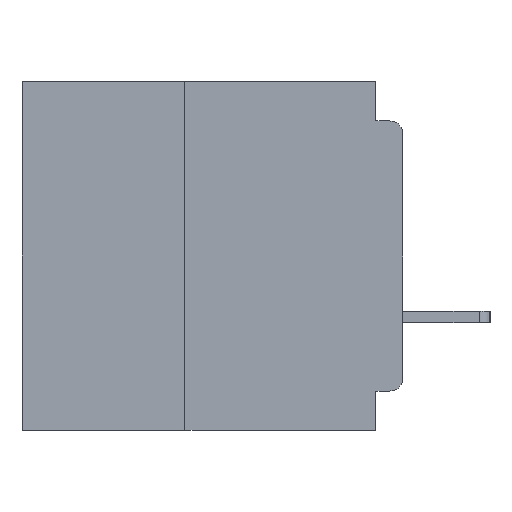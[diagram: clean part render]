
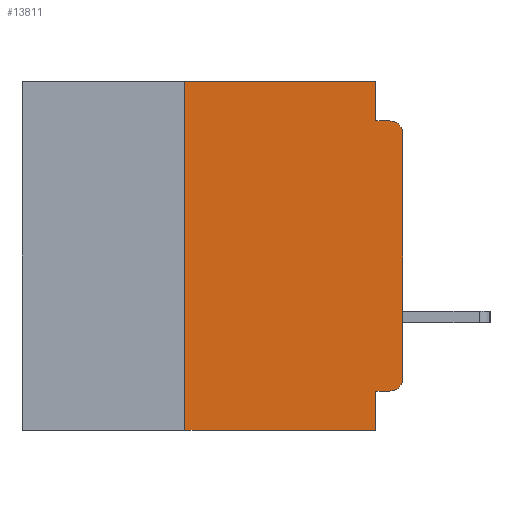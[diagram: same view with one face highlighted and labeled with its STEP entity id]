
A CAD part, left-side view. The second image highlights one B-rep face of the part: STEP entity #13811.
In plain terms, the highlighted planar face has unit normal (-1, 0, 0).
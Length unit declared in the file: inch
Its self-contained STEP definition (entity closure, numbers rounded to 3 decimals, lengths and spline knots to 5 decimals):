
#309 = EDGE_CURVE ( 'NONE', #36454, #38292, #2453, .T. ) ;
#1928 = LINE ( 'NONE', #43107, #9298 ) ;
#2356 = CARTESIAN_POINT ( 'NONE',  ( 0., 0.031, 0. ) ) ;
#2453 = LINE ( 'NONE', #35825, #27884 ) ;
#3500 = DIRECTION ( 'NONE',  ( 0., 0., 1. ) ) ;
#4695 = ORIENTED_EDGE ( 'NONE', *, *, #309, .F. ) ;
#4948 = AXIS2_PLACEMENT_3D ( 'NONE', #11540, #36747, #15153 ) ;
#6119 = AXIS2_PLACEMENT_3D ( 'NONE', #19516, #44719, #23129 ) ;
#6169 = LINE ( 'NONE', #45189, #42315 ) ;
#8141 = CARTESIAN_POINT ( 'NONE',  ( 0., 0.437, -0.4 ) ) ;
#8371 = CARTESIAN_POINT ( 'NONE',  ( 0., 0.031, 0. ) ) ;
#8539 = VECTOR ( 'NONE', #34878, 39.37008 ) ;
#8747 = LINE ( 'NONE', #31282, #17254 ) ;
#9298 = VECTOR ( 'NONE', #3500, 39.37008 ) ;
#9347 = CARTESIAN_POINT ( 'NONE',  ( 0., 0.031, -0.045 ) ) ;
#10352 = LINE ( 'NONE', #8141, #28379 ) ;
#11044 = ORIENTED_EDGE ( 'NONE', *, *, #30380, .T. ) ;
#11198 = EDGE_CURVE ( 'NONE', #35608, #17319, #27740, .T. ) ;
#11540 = CARTESIAN_POINT ( 'NONE',  ( 0., 0.015, -0.06 ) ) ;
#11821 = DIRECTION ( 'NONE',  ( 0., -1., 0. ) ) ;
#12366 = EDGE_LOOP ( 'NONE', ( #11044, #24002, #21811, #13815, #34124, #15558, #24963, #35182, #4695, #12725 ) ) ;
#12725 = ORIENTED_EDGE ( 'NONE', *, *, #41138, .T. ) ;
#13356 = DIRECTION ( 'NONE',  ( 0., -1., 0. ) ) ;
#13811 = ADVANCED_FACE ( 'NONE', ( #39879 ), #14224, .F. ) ;
#13815 = ORIENTED_EDGE ( 'NONE', *, *, #11198, .F. ) ;
#14224 = PLANE ( 'NONE',  #33964 ) ;
#14741 = CIRCLE ( 'NONE', #4948, 0.015 ) ;
#15153 = DIRECTION ( 'NONE',  ( 0., 0., -1. ) ) ;
#15558 = ORIENTED_EDGE ( 'NONE', *, *, #16684, .F. ) ;
#16469 = EDGE_CURVE ( 'NONE', #34442, #16898, #10352, .T. ) ;
#16545 = CIRCLE ( 'NONE', #6119, 0.015 ) ;
#16684 = EDGE_CURVE ( 'NONE', #34442, #17549, #6169, .T. ) ;
#16898 = VERTEX_POINT ( 'NONE', #31930 ) ;
#17254 = VECTOR ( 'NONE', #13356, 39.37008 ) ;
#17319 = VERTEX_POINT ( 'NONE', #9347 ) ;
#17549 = VERTEX_POINT ( 'NONE', #28563 ) ;
#17862 = DIRECTION ( 'NONE',  ( 0., 0., -1. ) ) ;
#18451 = VECTOR ( 'NONE', #18762, 39.37008 ) ;
#18762 = DIRECTION ( 'NONE',  ( 0., 0., -1. ) ) ;
#19140 = VECTOR ( 'NONE', #30762, 39.37008 ) ;
#19516 = CARTESIAN_POINT ( 'NONE',  ( 0., 0.015, -0.34 ) ) ;
#19777 = VERTEX_POINT ( 'NONE', #31505 ) ;
#21811 = ORIENTED_EDGE ( 'NONE', *, *, #30209, .F. ) ;
#22001 = VERTEX_POINT ( 'NONE', #29022 ) ;
#23129 = DIRECTION ( 'NONE',  ( 0., 0., -1. ) ) ;
#24002 = ORIENTED_EDGE ( 'NONE', *, *, #42208, .T. ) ;
#24963 = ORIENTED_EDGE ( 'NONE', *, *, #16469, .T. ) ;
#27740 = LINE ( 'NONE', #2356, #8539 ) ;
#27884 = VECTOR ( 'NONE', #35764, 39.37008 ) ;
#28379 = VECTOR ( 'NONE', #11821, 39.37008 ) ;
#28563 = CARTESIAN_POINT ( 'NONE',  ( 0., 0.25, 0. ) ) ;
#29022 = CARTESIAN_POINT ( 'NONE',  ( 0., 0.015, -0.045 ) ) ;
#29978 = VERTEX_POINT ( 'NONE', #33659 ) ;
#30209 = EDGE_CURVE ( 'NONE', #17319, #22001, #8747, .T. ) ;
#30380 = EDGE_CURVE ( 'NONE', #19777, #29978, #1928, .T. ) ;
#30762 = DIRECTION ( 'NONE',  ( 0., -1., 0. ) ) ;
#31282 = CARTESIAN_POINT ( 'NONE',  ( 0., 0., -0.045 ) ) ;
#31505 = CARTESIAN_POINT ( 'NONE',  ( 0., 0., -0.34 ) ) ;
#31930 = CARTESIAN_POINT ( 'NONE',  ( 0., 0.031, -0.4 ) ) ;
#33072 = CARTESIAN_POINT ( 'NONE',  ( 0., 0.031, -0.4 ) ) ;
#33554 = EDGE_CURVE ( 'NONE', #17549, #35608, #46719, .T. ) ;
#33659 = CARTESIAN_POINT ( 'NONE',  ( 0., 0., -0.06 ) ) ;
#33964 = AXIS2_PLACEMENT_3D ( 'NONE', #35807, #39428, #17862 ) ;
#34124 = ORIENTED_EDGE ( 'NONE', *, *, #33554, .F. ) ;
#34395 = CARTESIAN_POINT ( 'NONE',  ( 0., 0.437, 0. ) ) ;
#34442 = VERTEX_POINT ( 'NONE', #43658 ) ;
#34462 = DIRECTION ( 'NONE',  ( 0., 0., 1. ) ) ;
#34878 = DIRECTION ( 'NONE',  ( 0., 0., -1. ) ) ;
#35182 = ORIENTED_EDGE ( 'NONE', *, *, #36215, .F. ) ;
#35608 = VERTEX_POINT ( 'NONE', #8371 ) ;
#35764 = DIRECTION ( 'NONE',  ( 0., 1., 0. ) ) ;
#35807 = CARTESIAN_POINT ( 'NONE',  ( 0., 0.437, 0. ) ) ;
#35825 = CARTESIAN_POINT ( 'NONE',  ( 0., 0., -0.355 ) ) ;
#36215 = EDGE_CURVE ( 'NONE', #38292, #16898, #37631, .T. ) ;
#36454 = VERTEX_POINT ( 'NONE', #41751 ) ;
#36747 = DIRECTION ( 'NONE',  ( -1., 0., 0. ) ) ;
#37631 = LINE ( 'NONE', #33072, #18451 ) ;
#38292 = VERTEX_POINT ( 'NONE', #45977 ) ;
#39428 = DIRECTION ( 'NONE',  ( 1., 0., 0. ) ) ;
#39879 = FACE_OUTER_BOUND ( 'NONE', #12366, .T. ) ;
#41138 = EDGE_CURVE ( 'NONE', #36454, #19777, #16545, .T. ) ;
#41751 = CARTESIAN_POINT ( 'NONE',  ( 0., 0.015, -0.355 ) ) ;
#42208 = EDGE_CURVE ( 'NONE', #29978, #22001, #14741, .T. ) ;
#42315 = VECTOR ( 'NONE', #34462, 39.37008 ) ;
#43107 = CARTESIAN_POINT ( 'NONE',  ( 0., 0., 0. ) ) ;
#43658 = CARTESIAN_POINT ( 'NONE',  ( 0., 0.25, -0.4 ) ) ;
#44719 = DIRECTION ( 'NONE',  ( -1., 0., 0. ) ) ;
#45189 = CARTESIAN_POINT ( 'NONE',  ( 0., 0.25, -0.4 ) ) ;
#45977 = CARTESIAN_POINT ( 'NONE',  ( 0., 0.031, -0.355 ) ) ;
#46719 = LINE ( 'NONE', #34395, #19140 ) ;
